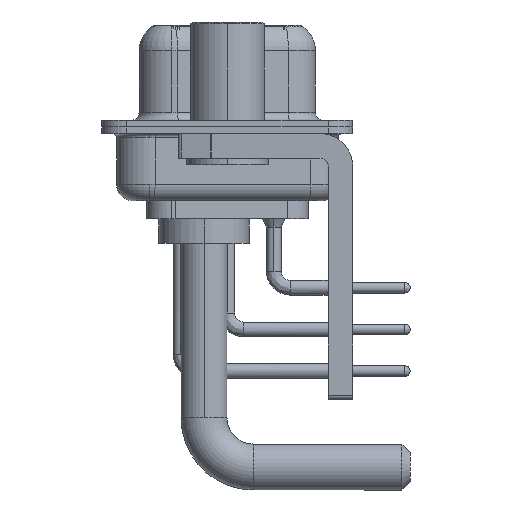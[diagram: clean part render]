
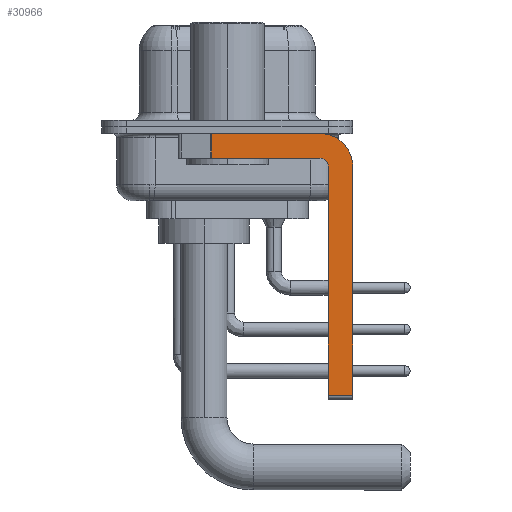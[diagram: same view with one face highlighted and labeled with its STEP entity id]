
A CAD part, left-side view. The second image highlights one B-rep face of the part: STEP entity #30966.
In plain terms, the highlighted planar face has unit normal (-1, 0, 0).
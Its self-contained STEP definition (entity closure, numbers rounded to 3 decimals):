
#280 = ORIENTED_EDGE ( 'NONE', *, *, #31292, .F. ) ;
#433 = CIRCLE ( 'NONE', #11790, 0.5 ) ;
#903 = ORIENTED_EDGE ( 'NONE', *, *, #18787, .F. ) ;
#2077 = VERTEX_POINT ( 'NONE', #13908 ) ;
#2093 = CARTESIAN_POINT ( 'NONE',  ( -2.9, 3., -0.4 ) ) ;
#3083 = DIRECTION ( 'NONE',  ( 0., 0., 1. ) ) ;
#3448 = VECTOR ( 'NONE', #21015, 1000. ) ;
#4401 = ORIENTED_EDGE ( 'NONE', *, *, #20510, .F. ) ;
#4937 = CARTESIAN_POINT ( 'NONE',  ( -2.9, -5.65, -16.35 ) ) ;
#5041 = VERTEX_POINT ( 'NONE', #30391 ) ;
#5142 = CARTESIAN_POINT ( 'NONE',  ( -2.9, -5.65, -1.9 ) ) ;
#6098 = EDGE_CURVE ( 'NONE', #2077, #27392, #433, .T. ) ;
#6124 = DIRECTION ( 'NONE',  ( 0., 1., 0. ) ) ;
#6846 = VERTEX_POINT ( 'NONE', #7713 ) ;
#7713 = CARTESIAN_POINT ( 'NONE',  ( -2.9, -6.15, -16.35 ) ) ;
#7730 = EDGE_CURVE ( 'NONE', #15533, #12186, #11643, .T. ) ;
#8726 = VERTEX_POINT ( 'NONE', #29753 ) ;
#8972 = CARTESIAN_POINT ( 'NONE',  ( -2.9, 0.978, -0.4 ) ) ;
#8973 = CARTESIAN_POINT ( 'NONE',  ( -2.9, -7.65, -16.35 ) ) ;
#9182 = VECTOR ( 'NONE', #6124, 1000. ) ;
#9295 = CARTESIAN_POINT ( 'NONE',  ( -2.9, -5.65, -0.4 ) ) ;
#9315 = VECTOR ( 'NONE', #13883, 1000. ) ;
#9328 = LINE ( 'NONE', #4937, #29885 ) ;
#9823 = DIRECTION ( 'NONE',  ( 1., 0., 0. ) ) ;
#10078 = CIRCLE ( 'NONE', #28089, 2. ) ;
#10560 = CARTESIAN_POINT ( 'NONE',  ( -2.9, -5.65, -2.4 ) ) ;
#11156 = LINE ( 'NONE', #28091, #3448 ) ;
#11592 = ORIENTED_EDGE ( 'NONE', *, *, #18138, .F. ) ;
#11643 = LINE ( 'NONE', #2093, #30629 ) ;
#11790 = AXIS2_PLACEMENT_3D ( 'NONE', #27149, #12777, #3083 ) ;
#12186 = VERTEX_POINT ( 'NONE', #9295 ) ;
#12777 = DIRECTION ( 'NONE',  ( -1., 0., 0. ) ) ;
#13172 = ORIENTED_EDGE ( 'NONE', *, *, #7730, .F. ) ;
#13813 = EDGE_CURVE ( 'NONE', #6846, #23503, #9328, .T. ) ;
#13883 = DIRECTION ( 'NONE',  ( 0., 0., -1. ) ) ;
#13908 = CARTESIAN_POINT ( 'NONE',  ( -2.9, -6.15, -2.4 ) ) ;
#14824 = DIRECTION ( 'NONE',  ( 1., 0., 0. ) ) ;
#15264 = CARTESIAN_POINT ( 'NONE',  ( -2.9, -6.15, -16.6 ) ) ;
#15533 = VERTEX_POINT ( 'NONE', #8972 ) ;
#16008 = LINE ( 'NONE', #24323, #9315 ) ;
#16514 = DIRECTION ( 'NONE',  ( 0., -1., 0. ) ) ;
#17413 = DIRECTION ( 'NONE',  ( 0., 0., -1. ) ) ;
#17690 = LINE ( 'NONE', #15264, #22510 ) ;
#17999 = FACE_OUTER_BOUND ( 'NONE', #27377, .T. ) ;
#18138 = EDGE_CURVE ( 'NONE', #6846, #2077, #17690, .T. ) ;
#18787 = EDGE_CURVE ( 'NONE', #5041, #23503, #11156, .T. ) ;
#19175 = DIRECTION ( 'NONE',  ( 0., -1., 0. ) ) ;
#19881 = AXIS2_PLACEMENT_3D ( 'NONE', #10560, #9823, #25417 ) ;
#20288 = ORIENTED_EDGE ( 'NONE', *, *, #23027, .T. ) ;
#20308 = CARTESIAN_POINT ( 'NONE',  ( -2.9, -5.65, -2.4 ) ) ;
#20510 = EDGE_CURVE ( 'NONE', #27392, #8726, #20674, .T. ) ;
#20674 = LINE ( 'NONE', #23557, #9182 ) ;
#21015 = DIRECTION ( 'NONE',  ( 0., 0., -1. ) ) ;
#22510 = VECTOR ( 'NONE', #22519, 1000. ) ;
#22519 = DIRECTION ( 'NONE',  ( 0., 0., 1. ) ) ;
#23027 = EDGE_CURVE ( 'NONE', #15533, #8726, #16008, .T. ) ;
#23452 = ORIENTED_EDGE ( 'NONE', *, *, #6098, .F. ) ;
#23503 = VERTEX_POINT ( 'NONE', #8973 ) ;
#23557 = CARTESIAN_POINT ( 'NONE',  ( -2.9, -5.65, -1.9 ) ) ;
#24323 = CARTESIAN_POINT ( 'NONE',  ( -2.9, 0.978, -1.9 ) ) ;
#25295 = ORIENTED_EDGE ( 'NONE', *, *, #13813, .T. ) ;
#25417 = DIRECTION ( 'NONE',  ( 0., 0., -1. ) ) ;
#27149 = CARTESIAN_POINT ( 'NONE',  ( -2.9, -5.65, -2.4 ) ) ;
#27377 = EDGE_LOOP ( 'NONE', ( #13172, #20288, #4401, #23452, #11592, #25295, #903, #280 ) ) ;
#27392 = VERTEX_POINT ( 'NONE', #5142 ) ;
#28089 = AXIS2_PLACEMENT_3D ( 'NONE', #20308, #14824, #17413 ) ;
#28091 = CARTESIAN_POINT ( 'NONE',  ( -2.9, -7.65, -2.4 ) ) ;
#29753 = CARTESIAN_POINT ( 'NONE',  ( -2.9, 0.978, -1.9 ) ) ;
#29885 = VECTOR ( 'NONE', #19175, 1000. ) ;
#30391 = CARTESIAN_POINT ( 'NONE',  ( -2.9, -7.65, -2.4 ) ) ;
#30521 = PLANE ( 'NONE',  #19881 ) ;
#30629 = VECTOR ( 'NONE', #16514, 1000. ) ;
#30966 = ADVANCED_FACE ( 'NONE', ( #17999 ), #30521, .F. ) ;
#31292 = EDGE_CURVE ( 'NONE', #12186, #5041, #10078, .T. ) ;
